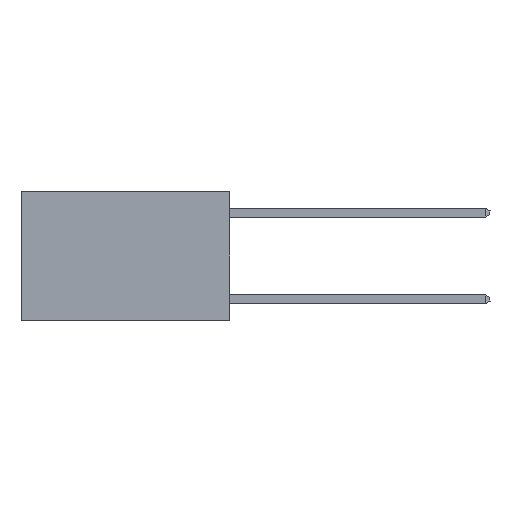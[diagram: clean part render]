
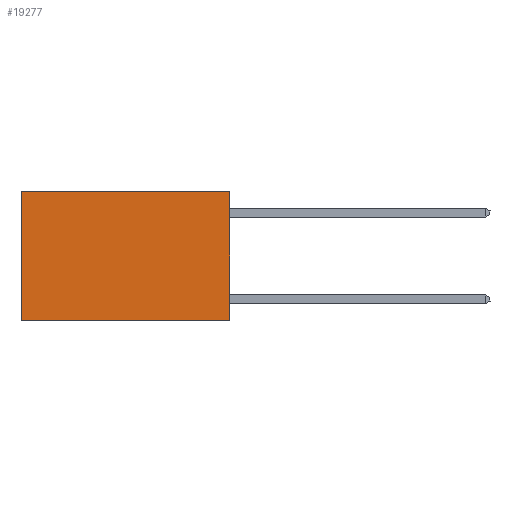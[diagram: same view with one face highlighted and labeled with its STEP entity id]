
A CAD part, left-side view. The second image highlights one B-rep face of the part: STEP entity #19277.
In plain terms, the highlighted planar face has unit normal (-1, 0, 0).
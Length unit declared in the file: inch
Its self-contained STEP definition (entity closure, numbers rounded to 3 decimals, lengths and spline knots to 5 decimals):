
#182 = DIRECTION ( 'NONE',  ( 0., 0., -1. ) ) ;
#2943 = CARTESIAN_POINT ( 'NONE',  ( 0.2625, 0.6, 0. ) ) ;
#4403 = DIRECTION ( 'NONE',  ( 1., 0., 0. ) ) ;
#4642 = VERTEX_POINT ( 'NONE', #11785 ) ;
#4979 = DIRECTION ( 'NONE',  ( 0., 0., -1. ) ) ;
#5986 = CARTESIAN_POINT ( 'NONE',  ( 0.2625, 0., -0.37 ) ) ;
#6391 = VECTOR ( 'NONE', #17595, 39.37008 ) ;
#8289 = VERTEX_POINT ( 'NONE', #19214 ) ;
#8752 = VECTOR ( 'NONE', #24402, 39.37008 ) ;
#9961 = CARTESIAN_POINT ( 'NONE',  ( 0.2625, 0., 0. ) ) ;
#11186 = EDGE_CURVE ( 'NONE', #21243, #13750, #12293, .T. ) ;
#11238 = DIRECTION ( 'NONE',  ( 0., 1., 0. ) ) ;
#11694 = CARTESIAN_POINT ( 'NONE',  ( 0.2625, 0., 0. ) ) ;
#11734 = FACE_OUTER_BOUND ( 'NONE', #20840, .T. ) ;
#11785 = CARTESIAN_POINT ( 'NONE',  ( 0.2625, 0.6, -0.37 ) ) ;
#12087 = LINE ( 'NONE', #12235, #8752 ) ;
#12235 = CARTESIAN_POINT ( 'NONE',  ( 0.2625, 0., -0.37 ) ) ;
#12293 = LINE ( 'NONE', #9961, #6391 ) ;
#13007 = ORIENTED_EDGE ( 'NONE', *, *, #11186, .F. ) ;
#13750 = VERTEX_POINT ( 'NONE', #5986 ) ;
#15628 = ORIENTED_EDGE ( 'NONE', *, *, #23052, .F. ) ;
#15922 = LINE ( 'NONE', #11694, #17366 ) ;
#17366 = VECTOR ( 'NONE', #11238, 39.37008 ) ;
#17595 = DIRECTION ( 'NONE',  ( 0., 0., -1. ) ) ;
#18277 = ORIENTED_EDGE ( 'NONE', *, *, #28632, .T. ) ;
#19214 = CARTESIAN_POINT ( 'NONE',  ( 0.2625, 0.6, 0. ) ) ;
#19277 = ADVANCED_FACE ( 'NONE', ( #11734 ), #21559, .F. ) ;
#19795 = CARTESIAN_POINT ( 'NONE',  ( 0.2625, 0., 0. ) ) ;
#20070 = AXIS2_PLACEMENT_3D ( 'NONE', #23294, #4403, #182 ) ;
#20840 = EDGE_LOOP ( 'NONE', ( #28702, #15628, #13007, #18277 ) ) ;
#21243 = VERTEX_POINT ( 'NONE', #19795 ) ;
#21559 = PLANE ( 'NONE',  #20070 ) ;
#23052 = EDGE_CURVE ( 'NONE', #13750, #4642, #12087, .T. ) ;
#23294 = CARTESIAN_POINT ( 'NONE',  ( 0.2625, 0., 0. ) ) ;
#23723 = VECTOR ( 'NONE', #4979, 39.37008 ) ;
#24180 = LINE ( 'NONE', #2943, #23723 ) ;
#24402 = DIRECTION ( 'NONE',  ( 0., 1., 0. ) ) ;
#25182 = EDGE_CURVE ( 'NONE', #8289, #4642, #24180, .T. ) ;
#28632 = EDGE_CURVE ( 'NONE', #21243, #8289, #15922, .T. ) ;
#28702 = ORIENTED_EDGE ( 'NONE', *, *, #25182, .T. ) ;
